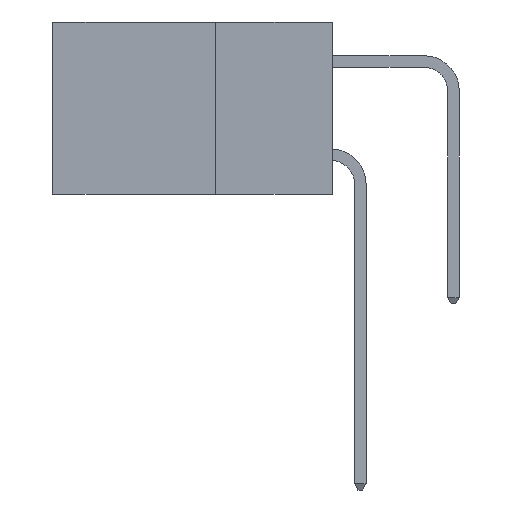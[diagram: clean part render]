
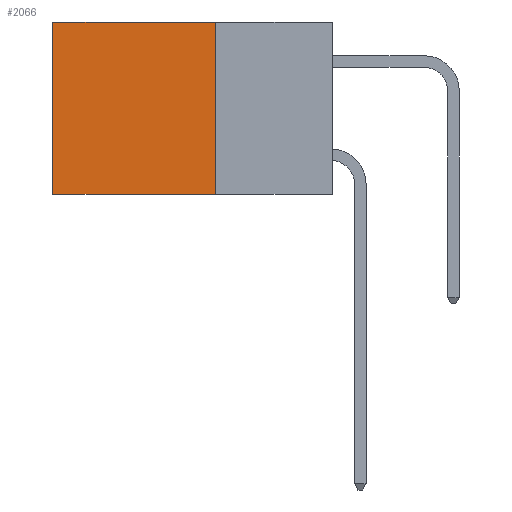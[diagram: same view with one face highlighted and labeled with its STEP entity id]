
A CAD part, left-side view. The second image highlights one B-rep face of the part: STEP entity #2066.
In plain terms, the highlighted planar face has unit normal (-1, 0, 0).
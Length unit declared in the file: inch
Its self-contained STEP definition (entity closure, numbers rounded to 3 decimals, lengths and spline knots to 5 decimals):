
#741 = VECTOR ( 'NONE', #17539, 39.37008 ) ;
#742 = EDGE_CURVE ( 'NONE', #15631, #16990, #6064, .T. ) ;
#933 = VERTEX_POINT ( 'NONE', #16124 ) ;
#1341 = LINE ( 'NONE', #6842, #6424 ) ;
#2066 = ADVANCED_FACE ( 'NONE', ( #6666 ), #13086, .F. ) ;
#2448 = CARTESIAN_POINT ( 'NONE',  ( 0.2615, 0.25, 0. ) ) ;
#2562 = VERTEX_POINT ( 'NONE', #11727 ) ;
#3023 = EDGE_LOOP ( 'NONE', ( #22091, #10250, #11114, #12362 ) ) ;
#5394 = VECTOR ( 'NONE', #15462, 39.37008 ) ;
#6055 = CARTESIAN_POINT ( 'NONE',  ( 0.2615, 0.6, -0.37 ) ) ;
#6064 = LINE ( 'NONE', #25523, #5394 ) ;
#6424 = VECTOR ( 'NONE', #17654, 39.37008 ) ;
#6666 = FACE_OUTER_BOUND ( 'NONE', #3023, .T. ) ;
#6842 = CARTESIAN_POINT ( 'NONE',  ( 0.2615, 0.25, -0.37 ) ) ;
#10210 = AXIS2_PLACEMENT_3D ( 'NONE', #13118, #13046, #13045 ) ;
#10250 = ORIENTED_EDGE ( 'NONE', *, *, #742, .F. ) ;
#11114 = ORIENTED_EDGE ( 'NONE', *, *, #12622, .F. ) ;
#11258 = EDGE_CURVE ( 'NONE', #933, #2562, #17279, .T. ) ;
#11727 = CARTESIAN_POINT ( 'NONE',  ( 0.2615, 0.6, 0. ) ) ;
#12362 = ORIENTED_EDGE ( 'NONE', *, *, #11258, .T. ) ;
#12622 = EDGE_CURVE ( 'NONE', #933, #15631, #1341, .T. ) ;
#13045 = DIRECTION ( 'NONE',  ( 0., 0., -1. ) ) ;
#13046 = DIRECTION ( 'NONE',  ( 1., 0., 0. ) ) ;
#13086 = PLANE ( 'NONE',  #10210 ) ;
#13118 = CARTESIAN_POINT ( 'NONE',  ( 0.2615, 0.25, -0.37 ) ) ;
#13293 = DIRECTION ( 'NONE',  ( 0., 0., -1. ) ) ;
#14874 = CARTESIAN_POINT ( 'NONE',  ( 0.2615, 0.25, -0.37 ) ) ;
#15462 = DIRECTION ( 'NONE',  ( 0., 1., 0. ) ) ;
#15631 = VERTEX_POINT ( 'NONE', #14874 ) ;
#16124 = CARTESIAN_POINT ( 'NONE',  ( 0.2615, 0.25, 0. ) ) ;
#16990 = VERTEX_POINT ( 'NONE', #6055 ) ;
#17279 = LINE ( 'NONE', #2448, #741 ) ;
#17287 = EDGE_CURVE ( 'NONE', #2562, #16990, #19429, .T. ) ;
#17539 = DIRECTION ( 'NONE',  ( 0., 1., 0. ) ) ;
#17654 = DIRECTION ( 'NONE',  ( 0., 0., -1. ) ) ;
#19429 = LINE ( 'NONE', #19783, #26437 ) ;
#19783 = CARTESIAN_POINT ( 'NONE',  ( 0.2615, 0.6, -0.37 ) ) ;
#22091 = ORIENTED_EDGE ( 'NONE', *, *, #17287, .T. ) ;
#25523 = CARTESIAN_POINT ( 'NONE',  ( 0.2615, 0.25, -0.37 ) ) ;
#26437 = VECTOR ( 'NONE', #13293, 39.37008 ) ;
